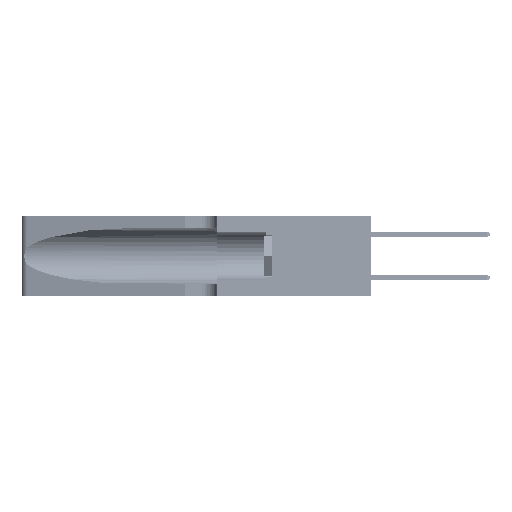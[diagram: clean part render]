
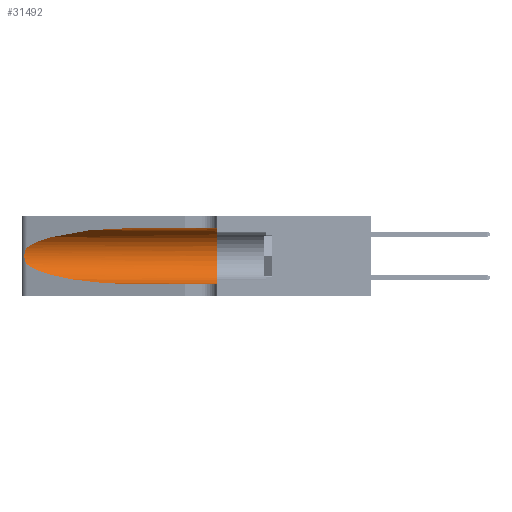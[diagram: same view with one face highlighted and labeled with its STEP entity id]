
A CAD part, left-side view. The second image highlights one B-rep face of the part: STEP entity #31492.
In plain terms, the highlighted cylindrical face has radius 3.308 mm (diameter 6.617 mm), a partial arc.
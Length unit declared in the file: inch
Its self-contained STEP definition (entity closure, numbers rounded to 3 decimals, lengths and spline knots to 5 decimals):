
#73 = CARTESIAN_POINT ( 'NONE',  ( 0.18966, 0.96281, 0.05475 ) ) ;
#195 = ORIENTED_EDGE ( 'NONE', *, *, #15235, .F. ) ;
#1131 = CARTESIAN_POINT ( 'NONE',  ( 0.25487, 1.22718, 0.22369 ) ) ;
#1670 = B_SPLINE_CURVE_WITH_KNOTS ( 'NONE', 3,
 ( #49973, #38329, #30339, #41732, #38158, #50149, #18930, #34362, #49487, #7390, #37983, #14877, #11325, #26774 ),
 .UNSPECIFIED., .F., .F.,
 ( 4, 2, 2, 2, 2, 2, 4 ),
 ( 0., 0.00027, 0.00053, 0.00107, 0.0016, 0.00187, 0.00214 ),
 .UNSPECIFIED. ) ;
#1797 = CARTESIAN_POINT ( 'NONE',  ( 0.25487, 1.22718, 0.14631 ) ) ;
#4101 = ORIENTED_EDGE ( 'NONE', *, *, #16074, .T. ) ;
#4451 = CARTESIAN_POINT ( 'NONE',  ( 0.25487, 1.22718, 0.14631 ) ) ;
#4489 = CARTESIAN_POINT ( 'NONE',  ( 0.1305, 1.61858, 0.185 ) ) ;
#4830 = FACE_OUTER_BOUND ( 'NONE', #34159, .T. ) ;
#5105 = EDGE_CURVE ( 'NONE', #17021, #43851, #18406, .T. ) ;
#5456 = LINE ( 'NONE', #49069, #7890 ) ;
#5959 = DIRECTION ( 'NONE',  ( 0., 1., 0. ) ) ;
#7390 = CARTESIAN_POINT ( 'NONE',  ( 0.25856, 1.23593, 0.16098 ) ) ;
#7523 = VERTEX_POINT ( 'NONE', #8891 ) ;
#7632 = CIRCLE ( 'NONE', #31957, 0.13025 ) ;
#7890 = VECTOR ( 'NONE', #33610, 39.37008 ) ;
#8573 = DIRECTION ( 'NONE',  ( 0., 0., -1. ) ) ;
#8891 = CARTESIAN_POINT ( 'NONE',  ( 0.1305, 0.35, 0.31525 ) ) ;
#11325 = CARTESIAN_POINT ( 'NONE',  ( 0.25555, 1.22993, 0.14849 ) ) ;
#12032 = CARTESIAN_POINT ( 'NONE',  ( 0.1305, 0.35, 0.05475 ) ) ;
#12177 = CYLINDRICAL_SURFACE ( 'NONE', #32830, 0.13025 ) ;
#14877 = CARTESIAN_POINT ( 'NONE',  ( 0.25639, 1.23186, 0.15144 ) ) ;
#15235 = EDGE_CURVE ( 'NONE', #18517, #7523, #5456, .T. ) ;
#15567 = CARTESIAN_POINT ( 'NONE',  ( 0.25487, 1.22718, 0.22369 ) ) ;
#15892 = CARTESIAN_POINT ( 'NONE',  ( 0.18966, 0.96281, 0.31525 ) ) ;
#16074 = EDGE_CURVE ( 'NONE', #27442, #36482, #1670, .T. ) ;
#16788 = EDGE_CURVE ( 'NONE', #36482, #17021, #24999, .T. ) ;
#17021 = VERTEX_POINT ( 'NONE', #17693 ) ;
#17693 = CARTESIAN_POINT ( 'NONE',  ( 0.1305, 0.72297, 0.05475 ) ) ;
#18406 = LINE ( 'NONE', #44194, #38517 ) ;
#18517 = VERTEX_POINT ( 'NONE', #35175 ) ;
#18930 = CARTESIAN_POINT ( 'NONE',  ( 0.26075, 1.23896, 0.19203 ) ) ;
#19860 = EDGE_CURVE ( 'NONE', #18517, #27442, #49542, .T. ) ;
#20460 = DIRECTION ( 'NONE',  ( 0., -1., 0. ) ) ;
#24999 =( BOUNDED_CURVE ( )  B_SPLINE_CURVE ( 3, ( #4451, #47253, #73, #43018 ),
 .UNSPECIFIED., .F., .F. ) 
 B_SPLINE_CURVE_WITH_KNOTS ( ( 4, 4 ),
 ( 3.44316, 4.71239 ),
 .UNSPECIFIED. ) 
 CURVE ( )  GEOMETRIC_REPRESENTATION_ITEM ( )  RATIONAL_B_SPLINE_CURVE ( ( 1., 0.87, 0.87, 1. ) ) 
 REPRESENTATION_ITEM ( '' )  );
#26774 = CARTESIAN_POINT ( 'NONE',  ( 0.25487, 1.22718, 0.14631 ) ) ;
#27442 = VERTEX_POINT ( 'NONE', #1131 ) ;
#27461 = CARTESIAN_POINT ( 'NONE',  ( 0.1305, 0.72297, 0.31525 ) ) ;
#29247 = CARTESIAN_POINT ( 'NONE',  ( 0.1305, 0.35, 0.185 ) ) ;
#29308 = ORIENTED_EDGE ( 'NONE', *, *, #35103, .F. ) ;
#30339 = CARTESIAN_POINT ( 'NONE',  ( 0.25639, 1.23184, 0.21858 ) ) ;
#30457 = ORIENTED_EDGE ( 'NONE', *, *, #5105, .T. ) ;
#31492 = ADVANCED_FACE ( 'NONE', ( #4830 ), #12177, .F. ) ;
#31957 = AXIS2_PLACEMENT_3D ( 'NONE', #29247, #5959, #44371 ) ;
#32830 = AXIS2_PLACEMENT_3D ( 'NONE', #4489, #20460, #8573 ) ;
#33610 = DIRECTION ( 'NONE',  ( 0., -1., 0. ) ) ;
#34159 = EDGE_LOOP ( 'NONE', ( #42828, #4101, #35216, #30457, #29308, #195 ) ) ;
#34362 = CARTESIAN_POINT ( 'NONE',  ( 0.26075, 1.23896, 0.178 ) ) ;
#34743 = DIRECTION ( 'NONE',  ( 0., -1., 0. ) ) ;
#35103 = EDGE_CURVE ( 'NONE', #7523, #43851, #7632, .T. ) ;
#35175 = CARTESIAN_POINT ( 'NONE',  ( 0.1305, 0.72297, 0.31525 ) ) ;
#35216 = ORIENTED_EDGE ( 'NONE', *, *, #16788, .T. ) ;
#36482 = VERTEX_POINT ( 'NONE', #1797 ) ;
#37983 = CARTESIAN_POINT ( 'NONE',  ( 0.25789, 1.23486, 0.15765 ) ) ;
#38158 = CARTESIAN_POINT ( 'NONE',  ( 0.25854, 1.2359, 0.20912 ) ) ;
#38329 = CARTESIAN_POINT ( 'NONE',  ( 0.25555, 1.22994, 0.2215 ) ) ;
#38517 = VECTOR ( 'NONE', #34743, 39.37008 ) ;
#41732 = CARTESIAN_POINT ( 'NONE',  ( 0.25787, 1.23484, 0.2124 ) ) ;
#42828 = ORIENTED_EDGE ( 'NONE', *, *, #19860, .T. ) ;
#43018 = CARTESIAN_POINT ( 'NONE',  ( 0.1305, 0.72297, 0.05475 ) ) ;
#43851 = VERTEX_POINT ( 'NONE', #12032 ) ;
#44194 = CARTESIAN_POINT ( 'NONE',  ( 0.1305, 1.61858, 0.05475 ) ) ;
#44371 = DIRECTION ( 'NONE',  ( 0., 0., 1. ) ) ;
#46463 = CARTESIAN_POINT ( 'NONE',  ( 0.2373, 1.15595, 0.28018 ) ) ;
#47253 = CARTESIAN_POINT ( 'NONE',  ( 0.2373, 1.15595, 0.08982 ) ) ;
#49069 = CARTESIAN_POINT ( 'NONE',  ( 0.1305, 1.61858, 0.31525 ) ) ;
#49487 = CARTESIAN_POINT ( 'NONE',  ( 0.26017, 1.23833, 0.17102 ) ) ;
#49542 =( BOUNDED_CURVE ( )  B_SPLINE_CURVE ( 3, ( #27461, #15892, #46463, #15567 ),
 .UNSPECIFIED., .F., .F. ) 
 B_SPLINE_CURVE_WITH_KNOTS ( ( 4, 4 ),
 ( 1.5708, 2.84003 ),
 .UNSPECIFIED. ) 
 CURVE ( )  GEOMETRIC_REPRESENTATION_ITEM ( )  RATIONAL_B_SPLINE_CURVE ( ( 1., 0.87, 0.87, 1. ) ) 
 REPRESENTATION_ITEM ( '' )  );
#49973 = CARTESIAN_POINT ( 'NONE',  ( 0.25487, 1.22718, 0.22369 ) ) ;
#50149 = CARTESIAN_POINT ( 'NONE',  ( 0.26018, 1.23835, 0.19895 ) ) ;
